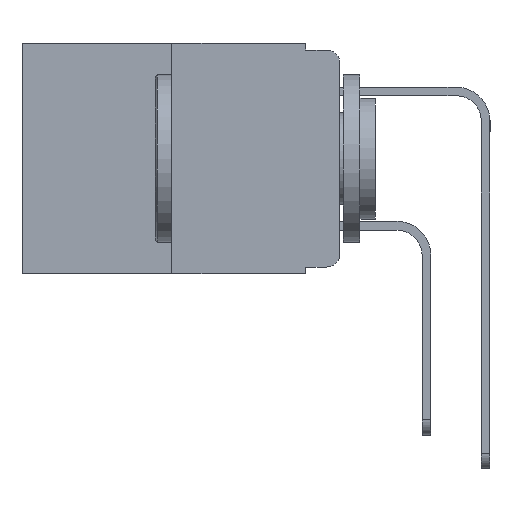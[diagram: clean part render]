
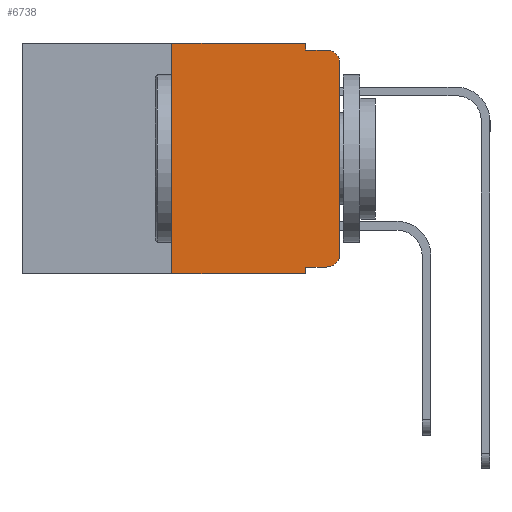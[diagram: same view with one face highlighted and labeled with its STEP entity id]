
A CAD part, left-side view. The second image highlights one B-rep face of the part: STEP entity #6738.
In plain terms, the highlighted planar face has unit normal (-1, 0, 0).
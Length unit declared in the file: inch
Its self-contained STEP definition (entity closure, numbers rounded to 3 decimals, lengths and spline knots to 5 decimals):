
#83 = VERTEX_POINT ( 'NONE', #3004 ) ;
#132 = CARTESIAN_POINT ( 'NONE',  ( 0., 0.051, -0.01 ) ) ;
#405 = VERTEX_POINT ( 'NONE', #8420 ) ;
#473 = CARTESIAN_POINT ( 'NONE',  ( 0., 0.051, 0. ) ) ;
#626 = EDGE_CURVE ( 'NONE', #7716, #405, #3462, .T. ) ;
#676 = DIRECTION ( 'NONE',  ( -1., 0., 0. ) ) ;
#695 = LINE ( 'NONE', #4676, #11140 ) ;
#868 = ORIENTED_EDGE ( 'NONE', *, *, #4415, .T. ) ;
#931 = DIRECTION ( 'NONE',  ( 0., 0., -1. ) ) ;
#960 = CARTESIAN_POINT ( 'NONE',  ( 0., 0.051, -0.333 ) ) ;
#1072 = DIRECTION ( 'NONE',  ( 0., 0., 1. ) ) ;
#1095 = CARTESIAN_POINT ( 'NONE',  ( 0., 0.25, 0. ) ) ;
#1138 = VECTOR ( 'NONE', #13090, 39.37008 ) ;
#1214 = CARTESIAN_POINT ( 'NONE',  ( 0., 0.051, -0.343 ) ) ;
#1502 = LINE ( 'NONE', #4942, #1138 ) ;
#1662 = VECTOR ( 'NONE', #3321, 39.37008 ) ;
#1787 = CARTESIAN_POINT ( 'NONE',  ( 0., 0.02, -0.03 ) ) ;
#1842 = VECTOR ( 'NONE', #9810, 39.37008 ) ;
#1853 = VERTEX_POINT ( 'NONE', #8430 ) ;
#2005 = CARTESIAN_POINT ( 'NONE',  ( 0., 0.473, 0. ) ) ;
#2124 = DIRECTION ( 'NONE',  ( 0., 0., 1. ) ) ;
#2192 = ORIENTED_EDGE ( 'NONE', *, *, #626, .T. ) ;
#2769 = VERTEX_POINT ( 'NONE', #473 ) ;
#2866 = EDGE_CURVE ( 'NONE', #9825, #3214, #695, .T. ) ;
#2976 = DIRECTION ( 'NONE',  ( 0., -1., 0. ) ) ;
#3004 = CARTESIAN_POINT ( 'NONE',  ( 0., 0., -0.313 ) ) ;
#3052 = DIRECTION ( 'NONE',  ( 0., 0., -1. ) ) ;
#3214 = VERTEX_POINT ( 'NONE', #1214 ) ;
#3305 = DIRECTION ( 'NONE',  ( 0., -1., 0. ) ) ;
#3321 = DIRECTION ( 'NONE',  ( 0., 0., -1. ) ) ;
#3462 = CIRCLE ( 'NONE', #4969, 0.02 ) ;
#3536 = CARTESIAN_POINT ( 'NONE',  ( 0., 0.25, -0.343 ) ) ;
#3635 = CARTESIAN_POINT ( 'NONE',  ( 0., 0.051, 0. ) ) ;
#3695 = CARTESIAN_POINT ( 'NONE',  ( 0., 0., -0.03 ) ) ;
#3801 = VERTEX_POINT ( 'NONE', #8121 ) ;
#4170 = ORIENTED_EDGE ( 'NONE', *, *, #2866, .T. ) ;
#4219 = VERTEX_POINT ( 'NONE', #132 ) ;
#4415 = EDGE_CURVE ( 'NONE', #83, #7716, #12204, .T. ) ;
#4598 = VECTOR ( 'NONE', #3305, 39.37008 ) ;
#4636 = DIRECTION ( 'NONE',  ( -1., 0., 0. ) ) ;
#4676 = CARTESIAN_POINT ( 'NONE',  ( 0., 0.473, -0.343 ) ) ;
#4942 = CARTESIAN_POINT ( 'NONE',  ( 0., 0.051, -0.01 ) ) ;
#4969 = AXIS2_PLACEMENT_3D ( 'NONE', #1787, #676, #931 ) ;
#5005 = LINE ( 'NONE', #1095, #7747 ) ;
#5109 = EDGE_CURVE ( 'NONE', #9825, #6038, #5005, .T. ) ;
#5560 = AXIS2_PLACEMENT_3D ( 'NONE', #10767, #4636, #11811 ) ;
#5908 = ORIENTED_EDGE ( 'NONE', *, *, #7034, .T. ) ;
#6038 = VERTEX_POINT ( 'NONE', #9098 ) ;
#6259 = ORIENTED_EDGE ( 'NONE', *, *, #12055, .F. ) ;
#6298 = ORIENTED_EDGE ( 'NONE', *, *, #12900, .F. ) ;
#6738 = ADVANCED_FACE ( 'NONE', ( #9440 ), #7183, .F. ) ;
#7034 = EDGE_CURVE ( 'NONE', #3801, #83, #11016, .T. ) ;
#7068 = EDGE_LOOP ( 'NONE', ( #868, #2192, #6259, #11545, #6298, #8387, #4170, #11428, #10819, #5908 ) ) ;
#7183 = PLANE ( 'NONE',  #8554 ) ;
#7314 = VECTOR ( 'NONE', #9336, 39.37008 ) ;
#7397 = CARTESIAN_POINT ( 'NONE',  ( 0., 0., 0. ) ) ;
#7544 = LINE ( 'NONE', #8501, #1662 ) ;
#7716 = VERTEX_POINT ( 'NONE', #3695 ) ;
#7747 = VECTOR ( 'NONE', #1072, 39.37008 ) ;
#8121 = CARTESIAN_POINT ( 'NONE',  ( 0., 0.02, -0.333 ) ) ;
#8387 = ORIENTED_EDGE ( 'NONE', *, *, #5109, .F. ) ;
#8410 = EDGE_CURVE ( 'NONE', #1853, #3801, #12691, .T. ) ;
#8420 = CARTESIAN_POINT ( 'NONE',  ( 0., 0.02, -0.01 ) ) ;
#8430 = CARTESIAN_POINT ( 'NONE',  ( 0., 0.051, -0.333 ) ) ;
#8501 = CARTESIAN_POINT ( 'NONE',  ( 0., 0.051, 0. ) ) ;
#8554 = AXIS2_PLACEMENT_3D ( 'NONE', #2005, #9253, #3052 ) ;
#9098 = CARTESIAN_POINT ( 'NONE',  ( 0., 0.25, 0. ) ) ;
#9253 = DIRECTION ( 'NONE',  ( 1., 0., 0. ) ) ;
#9336 = DIRECTION ( 'NONE',  ( 0., -1., 0. ) ) ;
#9440 = FACE_OUTER_BOUND ( 'NONE', #7068, .T. ) ;
#9810 = DIRECTION ( 'NONE',  ( 0., 0., -1. ) ) ;
#9825 = VERTEX_POINT ( 'NONE', #3536 ) ;
#10363 = LINE ( 'NONE', #13458, #4598 ) ;
#10767 = CARTESIAN_POINT ( 'NONE',  ( 0., 0.02, -0.313 ) ) ;
#10819 = ORIENTED_EDGE ( 'NONE', *, *, #8410, .T. ) ;
#11016 = CIRCLE ( 'NONE', #5560, 0.02 ) ;
#11140 = VECTOR ( 'NONE', #2976, 39.37008 ) ;
#11428 = ORIENTED_EDGE ( 'NONE', *, *, #12454, .F. ) ;
#11545 = ORIENTED_EDGE ( 'NONE', *, *, #12226, .F. ) ;
#11811 = DIRECTION ( 'NONE',  ( 0., 0., -1. ) ) ;
#12055 = EDGE_CURVE ( 'NONE', #4219, #405, #1502, .T. ) ;
#12204 = LINE ( 'NONE', #7397, #12827 ) ;
#12226 = EDGE_CURVE ( 'NONE', #2769, #4219, #7544, .T. ) ;
#12439 = LINE ( 'NONE', #3635, #1842 ) ;
#12454 = EDGE_CURVE ( 'NONE', #1853, #3214, #12439, .T. ) ;
#12691 = LINE ( 'NONE', #960, #7314 ) ;
#12827 = VECTOR ( 'NONE', #2124, 39.37008 ) ;
#12900 = EDGE_CURVE ( 'NONE', #6038, #2769, #10363, .T. ) ;
#13090 = DIRECTION ( 'NONE',  ( 0., -1., 0. ) ) ;
#13458 = CARTESIAN_POINT ( 'NONE',  ( 0., 0.473, 0. ) ) ;
